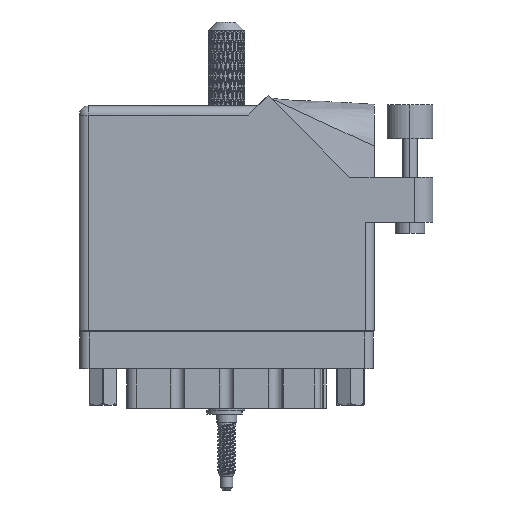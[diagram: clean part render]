
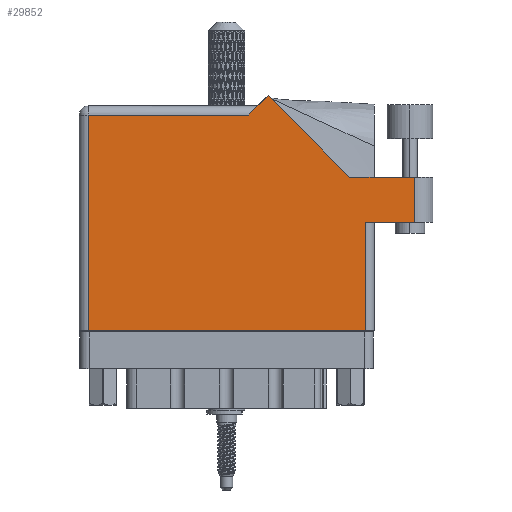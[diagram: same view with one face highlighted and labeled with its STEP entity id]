
A CAD part, front view. The second image highlights one B-rep face of the part: STEP entity #29852.
In plain terms, the highlighted face is planar.
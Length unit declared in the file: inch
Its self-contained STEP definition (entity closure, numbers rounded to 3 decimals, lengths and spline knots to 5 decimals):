
#2456 = EDGE_CURVE ( 'NONE', #21279, #60814, #58899, .T. ) ;
#3132 = ORIENTED_EDGE ( 'NONE', *, *, #56713, .T. ) ;
#5971 = VECTOR ( 'NONE', #75059, 39.37008 ) ;
#6763 = ORIENTED_EDGE ( 'NONE', *, *, #87085, .T. ) ;
#7547 = CARTESIAN_POINT ( 'NONE',  ( 2.41, 1.044, 0. ) ) ;
#10181 = VERTEX_POINT ( 'NONE', #80103 ) ;
#11208 = LINE ( 'NONE', #7547, #54511 ) ;
#11826 = AXIS2_PLACEMENT_3D ( 'NONE', #46763, #100650, #109257 ) ;
#14975 = DIRECTION ( 'NONE',  ( 0., 1., 0. ) ) ;
#15670 = ORIENTED_EDGE ( 'NONE', *, *, #15699, .T. ) ;
#15699 = EDGE_CURVE ( 'NONE', #60814, #96251, #82029, .T. ) ;
#18476 = EDGE_LOOP ( 'NONE', ( #3132, #44775, #56714, #21387, #15670, #63501, #96236, #93661, #6763 ) ) ;
#20656 = PLANE ( 'NONE',  #11826 ) ;
#20671 = CARTESIAN_POINT ( 'NONE',  ( 0., 0., 0. ) ) ;
#20721 = DIRECTION ( 'NONE',  ( 0., -1., 0. ) ) ;
#20909 = CARTESIAN_POINT ( 'NONE',  ( 2.01, 0.737, 0. ) ) ;
#21243 = VECTOR ( 'NONE', #90337, 39.37008 ) ;
#21279 = VERTEX_POINT ( 'NONE', #23535 ) ;
#21387 = ORIENTED_EDGE ( 'NONE', *, *, #2456, .T. ) ;
#21815 = CARTESIAN_POINT ( 'NONE',  ( 0., 1.468, 0. ) ) ;
#23535 = CARTESIAN_POINT ( 'NONE',  ( 1.84442, 1.044, 0. ) ) ;
#29852 = ADVANCED_FACE ( 'NONE', ( #102662 ), #20656, .F. ) ;
#33961 = CARTESIAN_POINT ( 'NONE',  ( 0.062, 0., 0. ) ) ;
#35137 = VERTEX_POINT ( 'NONE', #46496 ) ;
#35328 = VERTEX_POINT ( 'NONE', #33961 ) ;
#36104 = VECTOR ( 'NONE', #48713, 39.37008 ) ;
#37431 = DIRECTION ( 'NONE',  ( 0., 1., 0. ) ) ;
#38402 = LINE ( 'NONE', #68743, #78871 ) ;
#38611 = LINE ( 'NONE', #20671, #63739 ) ;
#39715 = EDGE_CURVE ( 'NONE', #35137, #35328, #113498, .T. ) ;
#44775 = ORIENTED_EDGE ( 'NONE', *, *, #103633, .T. ) ;
#46161 = EDGE_CURVE ( 'NONE', #35328, #73161, #38611, .T. ) ;
#46496 = CARTESIAN_POINT ( 'NONE',  ( 0.062, 1.468, 0. ) ) ;
#46763 = CARTESIAN_POINT ( 'NONE',  ( 0., 1.53, 0. ) ) ;
#48713 = DIRECTION ( 'NONE',  ( -1., 0., 0. ) ) ;
#49339 = CARTESIAN_POINT ( 'NONE',  ( 1.155, 1.468, 0. ) ) ;
#53767 = CARTESIAN_POINT ( 'NONE',  ( 1.217, 1.53, 0. ) ) ;
#54511 = VECTOR ( 'NONE', #69965, 39.37008 ) ;
#54601 = CARTESIAN_POINT ( 'NONE',  ( 2.285, 1.044, 0. ) ) ;
#55788 = CARTESIAN_POINT ( 'NONE',  ( 0.062, 0., 0. ) ) ;
#56527 = DIRECTION ( 'NONE',  ( 1., 0., 0. ) ) ;
#56713 = EDGE_CURVE ( 'NONE', #10181, #69239, #89764, .T. ) ;
#56714 = ORIENTED_EDGE ( 'NONE', *, *, #102555, .T. ) ;
#58899 = LINE ( 'NONE', #89965, #21243 ) ;
#60814 = VERTEX_POINT ( 'NONE', #113296 ) ;
#61120 = VECTOR ( 'NONE', #108062, 39.37008 ) ;
#61938 = VERTEX_POINT ( 'NONE', #99938 ) ;
#62798 = CARTESIAN_POINT ( 'NONE',  ( 2.285, 0.737, 0. ) ) ;
#63501 = ORIENTED_EDGE ( 'NONE', *, *, #105794, .T. ) ;
#63739 = VECTOR ( 'NONE', #56527, 39.37008 ) ;
#68743 = CARTESIAN_POINT ( 'NONE',  ( 1.948, 0.737, 0. ) ) ;
#69239 = VERTEX_POINT ( 'NONE', #62798 ) ;
#69965 = DIRECTION ( 'NONE',  ( -1., 0., 0. ) ) ;
#73161 = VERTEX_POINT ( 'NONE', #82985 ) ;
#75059 = DIRECTION ( 'NONE',  ( 1., 0., 0. ) ) ;
#78871 = VECTOR ( 'NONE', #14975, 39.37008 ) ;
#80103 = CARTESIAN_POINT ( 'NONE',  ( 1.948, 0.737, 0. ) ) ;
#82029 = LINE ( 'NONE', #53767, #61120 ) ;
#82985 = CARTESIAN_POINT ( 'NONE',  ( 1.948, 0., 0. ) ) ;
#87085 = EDGE_CURVE ( 'NONE', #73161, #10181, #38402, .T. ) ;
#89702 = VECTOR ( 'NONE', #20721, 39.37008 ) ;
#89764 = LINE ( 'NONE', #20909, #5971 ) ;
#89965 = CARTESIAN_POINT ( 'NONE',  ( 1.84442, 1.044, 0. ) ) ;
#90337 = DIRECTION ( 'NONE',  ( -0.707, 0.707, 0. ) ) ;
#93661 = ORIENTED_EDGE ( 'NONE', *, *, #46161, .T. ) ;
#96236 = ORIENTED_EDGE ( 'NONE', *, *, #39715, .T. ) ;
#96251 = VERTEX_POINT ( 'NONE', #49339 ) ;
#99938 = CARTESIAN_POINT ( 'NONE',  ( 2.285, 1.044, 0. ) ) ;
#100650 = DIRECTION ( 'NONE',  ( 0., 0., -1. ) ) ;
#102555 = EDGE_CURVE ( 'NONE', #61938, #21279, #11208, .T. ) ;
#102662 = FACE_OUTER_BOUND ( 'NONE', #18476, .T. ) ;
#103633 = EDGE_CURVE ( 'NONE', #69239, #61938, #107633, .T. ) ;
#105794 = EDGE_CURVE ( 'NONE', #96251, #35137, #107398, .T. ) ;
#107398 = LINE ( 'NONE', #21815, #36104 ) ;
#107633 = LINE ( 'NONE', #54601, #111788 ) ;
#108062 = DIRECTION ( 'NONE',  ( -0.707, -0.707, 0. ) ) ;
#109257 = DIRECTION ( 'NONE',  ( -1., 0., 0. ) ) ;
#111788 = VECTOR ( 'NONE', #37431, 39.37008 ) ;
#113296 = CARTESIAN_POINT ( 'NONE',  ( 1.28771, 1.60071, 0. ) ) ;
#113498 = LINE ( 'NONE', #55788, #89702 ) ;
